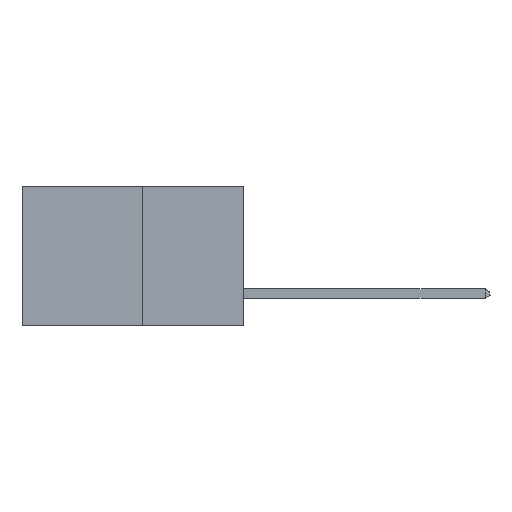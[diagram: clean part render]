
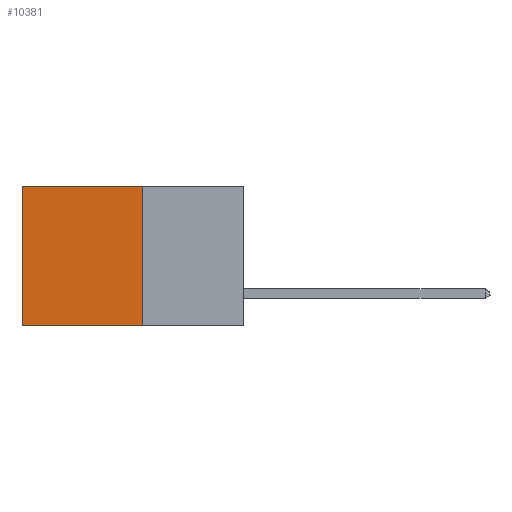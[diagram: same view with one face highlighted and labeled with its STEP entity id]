
A CAD part, left-side view. The second image highlights one B-rep face of the part: STEP entity #10381.
In plain terms, the highlighted planar face has unit normal (-1, 0, 0).
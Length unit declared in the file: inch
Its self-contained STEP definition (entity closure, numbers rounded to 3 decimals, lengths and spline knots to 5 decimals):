
#126 = CARTESIAN_POINT ( 'NONE',  ( 0.277, 0.59, 0. ) ) ;
#271 = VECTOR ( 'NONE', #9214, 39.37008 ) ;
#1668 = PLANE ( 'NONE',  #1888 ) ;
#1683 = ORIENTED_EDGE ( 'NONE', *, *, #8506, .T. ) ;
#1888 = AXIS2_PLACEMENT_3D ( 'NONE', #9439, #7744, #2544 ) ;
#2142 = DIRECTION ( 'NONE',  ( 0., 0., -1. ) ) ;
#2241 = ORIENTED_EDGE ( 'NONE', *, *, #9368, .F. ) ;
#2461 = VECTOR ( 'NONE', #2142, 39.37008 ) ;
#2544 = DIRECTION ( 'NONE',  ( 0., 0., -1. ) ) ;
#2591 = EDGE_CURVE ( 'NONE', #11060, #3561, #4912, .T. ) ;
#3251 = VERTEX_POINT ( 'NONE', #8005 ) ;
#3561 = VERTEX_POINT ( 'NONE', #4958 ) ;
#3825 = DIRECTION ( 'NONE',  ( 0., 1., 0. ) ) ;
#3947 = FACE_OUTER_BOUND ( 'NONE', #8848, .T. ) ;
#4033 = CARTESIAN_POINT ( 'NONE',  ( 0.277, 0.59, -0.37 ) ) ;
#4265 = CARTESIAN_POINT ( 'NONE',  ( 0.277, 0.27, 0. ) ) ;
#4786 = LINE ( 'NONE', #9089, #2461 ) ;
#4912 = LINE ( 'NONE', #4033, #271 ) ;
#4958 = CARTESIAN_POINT ( 'NONE',  ( 0.277, 0.59, -0.37 ) ) ;
#5248 = CARTESIAN_POINT ( 'NONE',  ( 0.277, 0.27, 0. ) ) ;
#5478 = ORIENTED_EDGE ( 'NONE', *, *, #2591, .T. ) ;
#5713 = EDGE_CURVE ( 'NONE', #8423, #3251, #4786, .T. ) ;
#6638 = ORIENTED_EDGE ( 'NONE', *, *, #5713, .F. ) ;
#7124 = LINE ( 'NONE', #10733, #9419 ) ;
#7408 = LINE ( 'NONE', #5248, #7685 ) ;
#7685 = VECTOR ( 'NONE', #7865, 39.37008 ) ;
#7744 = DIRECTION ( 'NONE',  ( 1., 0., 0. ) ) ;
#7865 = DIRECTION ( 'NONE',  ( 0., 1., 0. ) ) ;
#8005 = CARTESIAN_POINT ( 'NONE',  ( 0.277, 0.27, -0.37 ) ) ;
#8423 = VERTEX_POINT ( 'NONE', #4265 ) ;
#8506 = EDGE_CURVE ( 'NONE', #8423, #11060, #7408, .T. ) ;
#8848 = EDGE_LOOP ( 'NONE', ( #5478, #2241, #6638, #1683 ) ) ;
#9089 = CARTESIAN_POINT ( 'NONE',  ( 0.277, 0.27, -0.37 ) ) ;
#9214 = DIRECTION ( 'NONE',  ( 0., 0., -1. ) ) ;
#9368 = EDGE_CURVE ( 'NONE', #3251, #3561, #7124, .T. ) ;
#9419 = VECTOR ( 'NONE', #3825, 39.37008 ) ;
#9439 = CARTESIAN_POINT ( 'NONE',  ( 0.277, 0.27, -0.37 ) ) ;
#10381 = ADVANCED_FACE ( 'NONE', ( #3947 ), #1668, .F. ) ;
#10733 = CARTESIAN_POINT ( 'NONE',  ( 0.277, 0.27, -0.37 ) ) ;
#11060 = VERTEX_POINT ( 'NONE', #126 ) ;
